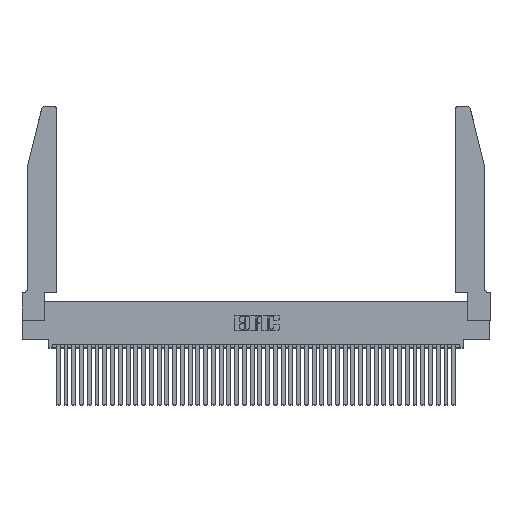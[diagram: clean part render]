
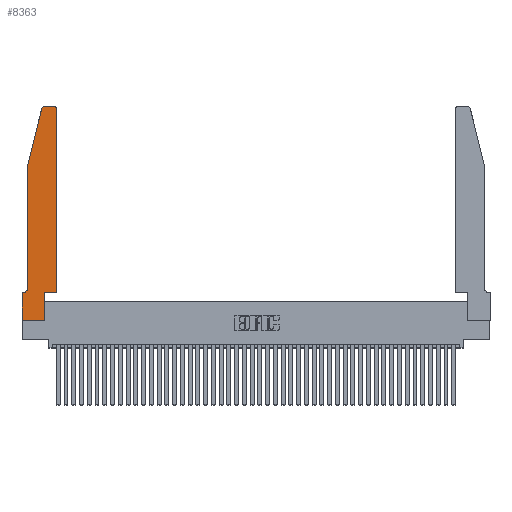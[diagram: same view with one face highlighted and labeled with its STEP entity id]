
A CAD part, top view. The second image highlights one B-rep face of the part: STEP entity #8363.
In plain terms, the highlighted planar face has unit normal (0, 0, 1).
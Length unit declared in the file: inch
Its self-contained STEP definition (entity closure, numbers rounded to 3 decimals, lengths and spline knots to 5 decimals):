
#366 = FACE_OUTER_BOUND ( 'NONE', #25081, .T. ) ;
#393 = DIRECTION ( 'NONE',  ( 0., -1., 0. ) ) ;
#932 = VERTEX_POINT ( 'NONE', #39082 ) ;
#1790 = AXIS2_PLACEMENT_3D ( 'NONE', #10978, #34662, #14448 ) ;
#3702 = DIRECTION ( 'NONE',  ( -0.239, -0.971, 0. ) ) ;
#4443 = CARTESIAN_POINT ( 'NONE',  ( 0.4505, 0.35, 0.37 ) ) ;
#4675 = CARTESIAN_POINT ( 'NONE',  ( 0.0755, 2., 0.37 ) ) ;
#4853 = DIRECTION ( 'NONE',  ( -1., 0., 0. ) ) ;
#5214 = VERTEX_POINT ( 'NONE', #14675 ) ;
#5413 = CARTESIAN_POINT ( 'NONE',  ( 0.284, 2.72, 0.37 ) ) ;
#5620 = CIRCLE ( 'NONE', #16838, 0.03 ) ;
#5766 = CARTESIAN_POINT ( 'NONE',  ( 0.4505, 0.35, 0.37 ) ) ;
#5918 = DIRECTION ( 'NONE',  ( 0., 1., 0. ) ) ;
#6587 = CARTESIAN_POINT ( 'NONE',  ( 0.4205, 2.75, 0.37 ) ) ;
#6819 = VERTEX_POINT ( 'NONE', #28367 ) ;
#7045 = CARTESIAN_POINT ( 'NONE',  ( 0.2605, 2.75, 0.37 ) ) ;
#7303 = ORIENTED_EDGE ( 'NONE', *, *, #33867, .T. ) ;
#7324 = EDGE_CURVE ( 'NONE', #17286, #5214, #40001, .T. ) ;
#8363 = ADVANCED_FACE ( 'NONE', ( #366 ), #16002, .T. ) ;
#8842 = VERTEX_POINT ( 'NONE', #36043 ) ;
#8926 = DIRECTION ( 'NONE',  ( 1., 0., 0. ) ) ;
#8955 = ORIENTED_EDGE ( 'NONE', *, *, #33123, .T. ) ;
#9496 = ORIENTED_EDGE ( 'NONE', *, *, #39846, .T. ) ;
#10188 = CARTESIAN_POINT ( 'NONE',  ( 0.4205, 2.72, 0.37 ) ) ;
#10978 = CARTESIAN_POINT ( 'NONE',  ( 0.0055, 0.42, 0.37 ) ) ;
#11466 = DIRECTION ( 'NONE',  ( 1., 0., 0. ) ) ;
#13314 = ORIENTED_EDGE ( 'NONE', *, *, #21831, .T. ) ;
#13537 = VECTOR ( 'NONE', #27646, 39.37008 ) ;
#13648 = DIRECTION ( 'NONE',  ( 1., 0., 0. ) ) ;
#13736 = LINE ( 'NONE', #4443, #38549 ) ;
#14079 = CARTESIAN_POINT ( 'NONE',  ( 0.0755, 2., 0.37 ) ) ;
#14448 = DIRECTION ( 'NONE',  ( -1., 0., 0. ) ) ;
#14675 = CARTESIAN_POINT ( 'NONE',  ( 0.2865, 0.35, 0.37 ) ) ;
#14695 = VERTEX_POINT ( 'NONE', #6587 ) ;
#14843 = EDGE_CURVE ( 'NONE', #8842, #29549, #30493, .T. ) ;
#16002 = PLANE ( 'NONE',  #41497 ) ;
#16548 = VERTEX_POINT ( 'NONE', #17178 ) ;
#16838 = AXIS2_PLACEMENT_3D ( 'NONE', #5413, #29315, #8926 ) ;
#16932 = CARTESIAN_POINT ( 'NONE',  ( 0.284, 2.75, 0.37 ) ) ;
#17178 = CARTESIAN_POINT ( 'NONE',  ( 0.4505, 2.72, 0.37 ) ) ;
#17286 = VERTEX_POINT ( 'NONE', #41509 ) ;
#18614 = CARTESIAN_POINT ( 'NONE',  ( 0.0755, 0.35, 0.37 ) ) ;
#19184 = ORIENTED_EDGE ( 'NONE', *, *, #25952, .T. ) ;
#19417 = DIRECTION ( 'NONE',  ( 1., 0., 0. ) ) ;
#20498 = VECTOR ( 'NONE', #393, 39.37008 ) ;
#21319 = ORIENTED_EDGE ( 'NONE', *, *, #38346, .T. ) ;
#21831 = EDGE_CURVE ( 'NONE', #16548, #14695, #43782, .T. ) ;
#22595 = LINE ( 'NONE', #7045, #13537 ) ;
#22755 = CARTESIAN_POINT ( 'NONE',  ( 0.4505, 0.35, 0.37 ) ) ;
#23797 = CARTESIAN_POINT ( 'NONE',  ( 0.0755, 2., 0.37 ) ) ;
#23956 = DIRECTION ( 'NONE',  ( 0., 1., 0. ) ) ;
#24405 = CARTESIAN_POINT ( 'NONE',  ( 0., 0., 0.37 ) ) ;
#24445 = ORIENTED_EDGE ( 'NONE', *, *, #25482, .T. ) ;
#24524 = VECTOR ( 'NONE', #4853, 39.37008 ) ;
#24771 = VECTOR ( 'NONE', #27169, 39.37008 ) ;
#25081 = EDGE_LOOP ( 'NONE', ( #41241, #24445, #7303, #35489, #9496, #38654, #32860, #8955, #27089, #19184, #21319, #13314 ) ) ;
#25482 = EDGE_CURVE ( 'NONE', #28161, #932, #5620, .T. ) ;
#25557 = VECTOR ( 'NONE', #5918, 39.37008 ) ;
#25952 = EDGE_CURVE ( 'NONE', #5214, #29845, #13736, .T. ) ;
#26019 = CARTESIAN_POINT ( 'NONE',  ( 0., 0.35, 0.37 ) ) ;
#27089 = ORIENTED_EDGE ( 'NONE', *, *, #7324, .T. ) ;
#27140 = LINE ( 'NONE', #23797, #28191 ) ;
#27154 = DIRECTION ( 'NONE',  ( 0., -1., 0. ) ) ;
#27169 = DIRECTION ( 'NONE',  ( 1., 0., 0. ) ) ;
#27646 = DIRECTION ( 'NONE',  ( -1., 0., 0. ) ) ;
#28161 = VERTEX_POINT ( 'NONE', #16932 ) ;
#28191 = VECTOR ( 'NONE', #27154, 39.37008 ) ;
#28367 = CARTESIAN_POINT ( 'NONE',  ( 0.0055, 0.35, 0.37 ) ) ;
#28892 = VECTOR ( 'NONE', #3702, 39.37008 ) ;
#29315 = DIRECTION ( 'NONE',  ( 0., 0., 1. ) ) ;
#29549 = VERTEX_POINT ( 'NONE', #34236 ) ;
#29677 = EDGE_CURVE ( 'NONE', #6819, #8842, #42391, .T. ) ;
#29845 = VERTEX_POINT ( 'NONE', #22755 ) ;
#30178 = CIRCLE ( 'NONE', #1790, 0.07 ) ;
#30493 = LINE ( 'NONE', #24405, #20498 ) ;
#30786 = CARTESIAN_POINT ( 'NONE',  ( 0.0755, 0.42, 0.37 ) ) ;
#31062 = VECTOR ( 'NONE', #23956, 39.37008 ) ;
#32829 = AXIS2_PLACEMENT_3D ( 'NONE', #10188, #33896, #13648 ) ;
#32860 = ORIENTED_EDGE ( 'NONE', *, *, #14843, .T. ) ;
#33123 = EDGE_CURVE ( 'NONE', #29549, #17286, #33709, .T. ) ;
#33709 = LINE ( 'NONE', #43915, #24771 ) ;
#33789 = CARTESIAN_POINT ( 'NONE',  ( 0.2865, 0.35, 0.37 ) ) ;
#33839 = VERTEX_POINT ( 'NONE', #30786 ) ;
#33867 = EDGE_CURVE ( 'NONE', #932, #35345, #37845, .T. ) ;
#33896 = DIRECTION ( 'NONE',  ( 0., 0., 1. ) ) ;
#34236 = CARTESIAN_POINT ( 'NONE',  ( 0., 0., 0.37 ) ) ;
#34500 = LINE ( 'NONE', #5766, #25557 ) ;
#34662 = DIRECTION ( 'NONE',  ( 0., 0., -1. ) ) ;
#35345 = VERTEX_POINT ( 'NONE', #4675 ) ;
#35489 = ORIENTED_EDGE ( 'NONE', *, *, #36625, .T. ) ;
#36043 = CARTESIAN_POINT ( 'NONE',  ( 0., 0.35, 0.37 ) ) ;
#36625 = EDGE_CURVE ( 'NONE', #35345, #33839, #27140, .T. ) ;
#37845 = LINE ( 'NONE', #14079, #28892 ) ;
#38346 = EDGE_CURVE ( 'NONE', #29845, #16548, #34500, .T. ) ;
#38549 = VECTOR ( 'NONE', #11466, 39.37008 ) ;
#38654 = ORIENTED_EDGE ( 'NONE', *, *, #29677, .T. ) ;
#39082 = CARTESIAN_POINT ( 'NONE',  ( 0.25487, 2.72718, 0.37 ) ) ;
#39570 = DIRECTION ( 'NONE',  ( 0., 0., 1. ) ) ;
#39846 = EDGE_CURVE ( 'NONE', #33839, #6819, #30178, .T. ) ;
#40001 = LINE ( 'NONE', #33789, #31062 ) ;
#41241 = ORIENTED_EDGE ( 'NONE', *, *, #42933, .T. ) ;
#41497 = AXIS2_PLACEMENT_3D ( 'NONE', #26019, #39570, #19417 ) ;
#41509 = CARTESIAN_POINT ( 'NONE',  ( 0.2865, 0., 0.37 ) ) ;
#42391 = LINE ( 'NONE', #18614, #24524 ) ;
#42933 = EDGE_CURVE ( 'NONE', #14695, #28161, #22595, .T. ) ;
#43782 = CIRCLE ( 'NONE', #32829, 0.03 ) ;
#43915 = CARTESIAN_POINT ( 'NONE',  ( 0., 0., 0.37 ) ) ;
